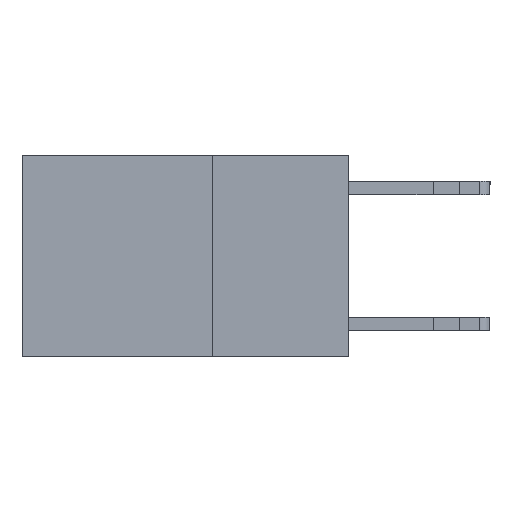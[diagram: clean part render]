
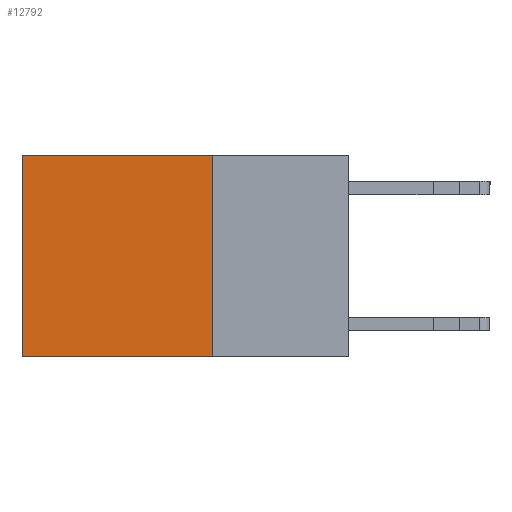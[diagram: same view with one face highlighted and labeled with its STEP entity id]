
A CAD part, left-side view. The second image highlights one B-rep face of the part: STEP entity #12792.
In plain terms, the highlighted planar face has unit normal (-1, 0, 0).
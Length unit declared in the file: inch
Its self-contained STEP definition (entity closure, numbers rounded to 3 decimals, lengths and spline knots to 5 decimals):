
#430 = AXIS2_PLACEMENT_3D ( 'NONE', #7007, #9136, #3952 ) ;
#993 = ORIENTED_EDGE ( 'NONE', *, *, #9880, .T. ) ;
#1025 = CARTESIAN_POINT ( 'NONE',  ( 0.2625, 0.25, 0. ) ) ;
#1819 = ORIENTED_EDGE ( 'NONE', *, *, #10468, .F. ) ;
#2100 = ORIENTED_EDGE ( 'NONE', *, *, #13179, .F. ) ;
#2176 = VERTEX_POINT ( 'NONE', #2198 ) ;
#2198 = CARTESIAN_POINT ( 'NONE',  ( 0.2625, 0.6, -0.37 ) ) ;
#2851 = PLANE ( 'NONE',  #430 ) ;
#3952 = DIRECTION ( 'NONE',  ( 0., 0., -1. ) ) ;
#4111 = DIRECTION ( 'NONE',  ( 0., 0., -1. ) ) ;
#4136 = VECTOR ( 'NONE', #6782, 39.37008 ) ;
#4614 = VECTOR ( 'NONE', #4111, 39.37008 ) ;
#4748 = ORIENTED_EDGE ( 'NONE', *, *, #9796, .T. ) ;
#5378 = VERTEX_POINT ( 'NONE', #10063 ) ;
#5394 = CARTESIAN_POINT ( 'NONE',  ( 0.2625, 0.25, -0.37 ) ) ;
#5959 = LINE ( 'NONE', #1025, #4614 ) ;
#6782 = DIRECTION ( 'NONE',  ( 0., 1., 0. ) ) ;
#7007 = CARTESIAN_POINT ( 'NONE',  ( 0.2625, 0.25, 0. ) ) ;
#7224 = EDGE_LOOP ( 'NONE', ( #993, #1819, #2100, #4748 ) ) ;
#7432 = CARTESIAN_POINT ( 'NONE',  ( 0.2625, 0.25, 0. ) ) ;
#7819 = CARTESIAN_POINT ( 'NONE',  ( 0.2625, 0.6, 0. ) ) ;
#7886 = DIRECTION ( 'NONE',  ( 0., 0., -1. ) ) ;
#7973 = CARTESIAN_POINT ( 'NONE',  ( 0.2625, 0.25, -0.37 ) ) ;
#8484 = LINE ( 'NONE', #5394, #10496 ) ;
#8845 = LINE ( 'NONE', #7819, #11359 ) ;
#8983 = CARTESIAN_POINT ( 'NONE',  ( 0.2625, 0.25, 0. ) ) ;
#9136 = DIRECTION ( 'NONE',  ( 1., 0., 0. ) ) ;
#9310 = DIRECTION ( 'NONE',  ( 0., 1., 0. ) ) ;
#9796 = EDGE_CURVE ( 'NONE', #11005, #5378, #13169, .T. ) ;
#9880 = EDGE_CURVE ( 'NONE', #5378, #2176, #8845, .T. ) ;
#10063 = CARTESIAN_POINT ( 'NONE',  ( 0.2625, 0.6, 0. ) ) ;
#10468 = EDGE_CURVE ( 'NONE', #12776, #2176, #8484, .T. ) ;
#10496 = VECTOR ( 'NONE', #9310, 39.37008 ) ;
#11005 = VERTEX_POINT ( 'NONE', #7432 ) ;
#11359 = VECTOR ( 'NONE', #7886, 39.37008 ) ;
#12224 = FACE_OUTER_BOUND ( 'NONE', #7224, .T. ) ;
#12776 = VERTEX_POINT ( 'NONE', #7973 ) ;
#12792 = ADVANCED_FACE ( 'NONE', ( #12224 ), #2851, .F. ) ;
#13169 = LINE ( 'NONE', #8983, #4136 ) ;
#13179 = EDGE_CURVE ( 'NONE', #11005, #12776, #5959, .T. ) ;
